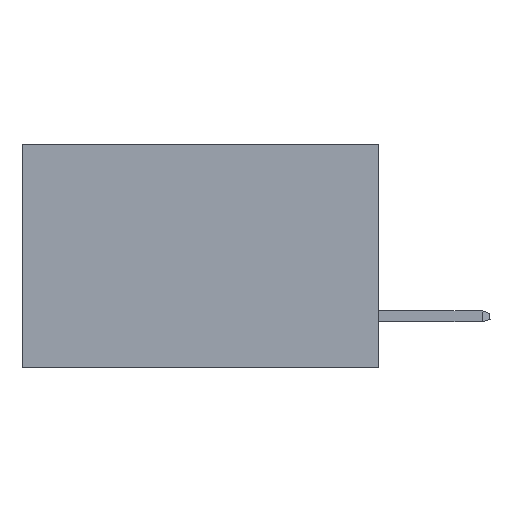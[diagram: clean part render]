
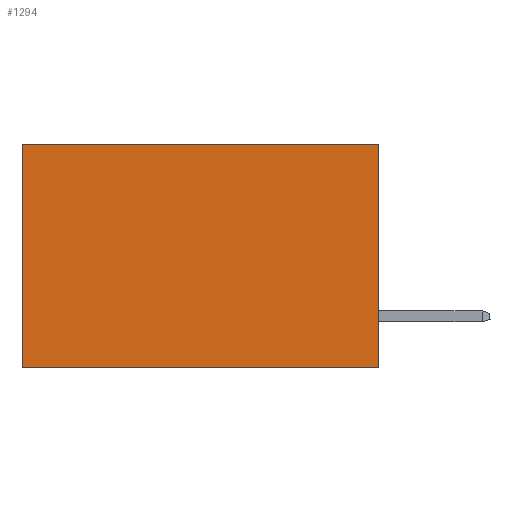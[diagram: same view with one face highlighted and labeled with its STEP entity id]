
A CAD part, left-side view. The second image highlights one B-rep face of the part: STEP entity #1294.
In plain terms, the highlighted planar face has unit normal (-1, 0, 0).
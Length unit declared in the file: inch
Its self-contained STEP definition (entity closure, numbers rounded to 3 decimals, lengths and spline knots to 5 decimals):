
#822 = LINE ( 'NONE', #25857, #25363 ) ;
#1294 = ADVANCED_FACE ( 'NONE', ( #24039 ), #16865, .F. ) ;
#2379 = CARTESIAN_POINT ( 'NONE',  ( 0.277, 0., -0.37 ) ) ;
#6050 = EDGE_LOOP ( 'NONE', ( #10007, #26922, #31256, #15298 ) ) ;
#6445 = DIRECTION ( 'NONE',  ( 0., 0., -1. ) ) ;
#7444 = DIRECTION ( 'NONE',  ( 0., 1., 0. ) ) ;
#9170 = EDGE_CURVE ( 'NONE', #20408, #12643, #22431, .T. ) ;
#9778 = EDGE_CURVE ( 'NONE', #27064, #20408, #12178, .T. ) ;
#10007 = ORIENTED_EDGE ( 'NONE', *, *, #31496, .T. ) ;
#12097 = DIRECTION ( 'NONE',  ( 0., 0., -1. ) ) ;
#12178 = LINE ( 'NONE', #19255, #29929 ) ;
#12643 = VERTEX_POINT ( 'NONE', #14696 ) ;
#13864 = DIRECTION ( 'NONE',  ( 0., 0., -1. ) ) ;
#13937 = DIRECTION ( 'NONE',  ( 1., 0., 0. ) ) ;
#14696 = CARTESIAN_POINT ( 'NONE',  ( 0.277, 0.59, -0.37 ) ) ;
#15298 = ORIENTED_EDGE ( 'NONE', *, *, #23622, .T. ) ;
#15927 = VECTOR ( 'NONE', #7444, 39.37008 ) ;
#16275 = AXIS2_PLACEMENT_3D ( 'NONE', #23908, #13937, #13864 ) ;
#16728 = LINE ( 'NONE', #22695, #22479 ) ;
#16865 = PLANE ( 'NONE',  #16275 ) ;
#19255 = CARTESIAN_POINT ( 'NONE',  ( 0.277, 0., -0.37 ) ) ;
#20408 = VERTEX_POINT ( 'NONE', #22813 ) ;
#21027 = CARTESIAN_POINT ( 'NONE',  ( 0.277, 0.59, 0. ) ) ;
#22431 = LINE ( 'NONE', #2379, #15927 ) ;
#22479 = VECTOR ( 'NONE', #25118, 39.37008 ) ;
#22695 = CARTESIAN_POINT ( 'NONE',  ( 0.277, 0., 0. ) ) ;
#22813 = CARTESIAN_POINT ( 'NONE',  ( 0.277, 0., -0.37 ) ) ;
#23622 = EDGE_CURVE ( 'NONE', #27064, #30942, #16728, .T. ) ;
#23908 = CARTESIAN_POINT ( 'NONE',  ( 0.277, 0., -0.37 ) ) ;
#24039 = FACE_OUTER_BOUND ( 'NONE', #6050, .T. ) ;
#25118 = DIRECTION ( 'NONE',  ( 0., 1., 0. ) ) ;
#25363 = VECTOR ( 'NONE', #6445, 39.37008 ) ;
#25857 = CARTESIAN_POINT ( 'NONE',  ( 0.277, 0.59, -0.37 ) ) ;
#26922 = ORIENTED_EDGE ( 'NONE', *, *, #9170, .F. ) ;
#27064 = VERTEX_POINT ( 'NONE', #30829 ) ;
#29929 = VECTOR ( 'NONE', #12097, 39.37008 ) ;
#30829 = CARTESIAN_POINT ( 'NONE',  ( 0.277, 0., 0. ) ) ;
#30942 = VERTEX_POINT ( 'NONE', #21027 ) ;
#31256 = ORIENTED_EDGE ( 'NONE', *, *, #9778, .F. ) ;
#31496 = EDGE_CURVE ( 'NONE', #30942, #12643, #822, .T. ) ;
